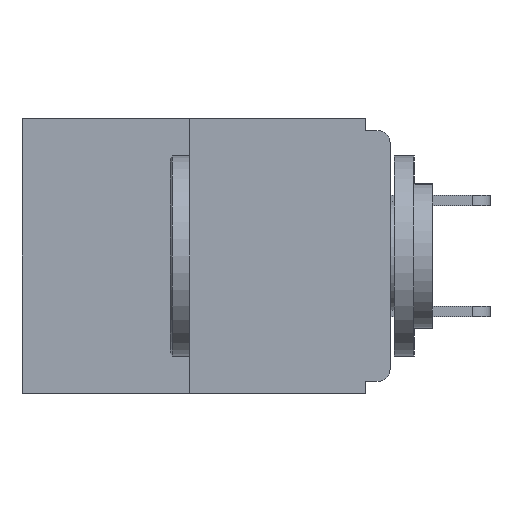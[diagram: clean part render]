
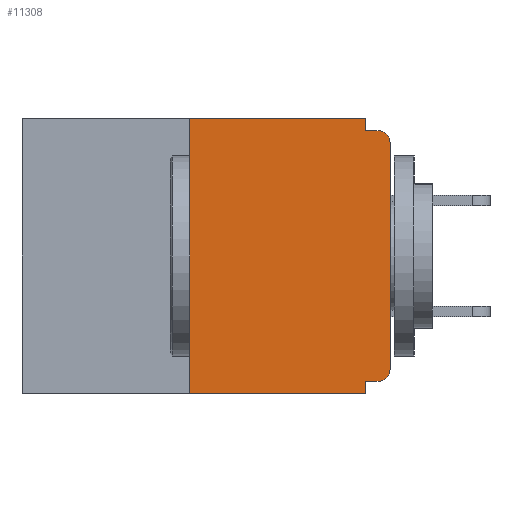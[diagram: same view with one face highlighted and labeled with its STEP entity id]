
A CAD part, left-side view. The second image highlights one B-rep face of the part: STEP entity #11308.
In plain terms, the highlighted planar face has unit normal (-1, 0, 0).
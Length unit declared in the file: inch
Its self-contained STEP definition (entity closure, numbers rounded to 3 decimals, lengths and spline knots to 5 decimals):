
#68 = CARTESIAN_POINT ( 'NONE',  ( 0., 0.25, 0. ) ) ;
#278 = CARTESIAN_POINT ( 'NONE',  ( 0., 0.031, -0.343 ) ) ;
#491 = DIRECTION ( 'NONE',  ( 0., 0., -1. ) ) ;
#777 = DIRECTION ( 'NONE',  ( 0., 0., -1. ) ) ;
#806 = LINE ( 'NONE', #7885, #6524 ) ;
#1189 = ORIENTED_EDGE ( 'NONE', *, *, #11605, .T. ) ;
#1291 = CARTESIAN_POINT ( 'NONE',  ( 0., 0.031, 0. ) ) ;
#1295 = CARTESIAN_POINT ( 'NONE',  ( 0., 0.031, -0.015 ) ) ;
#1330 = EDGE_CURVE ( 'NONE', #3055, #8899, #3673, .T. ) ;
#1400 = EDGE_CURVE ( 'NONE', #9018, #3647, #1813, .T. ) ;
#1755 = CARTESIAN_POINT ( 'NONE',  ( 0., 0.015, -0.328 ) ) ;
#1813 = LINE ( 'NONE', #68, #10220 ) ;
#2336 = DIRECTION ( 'NONE',  ( 0., 0., -1. ) ) ;
#2360 = AXIS2_PLACEMENT_3D ( 'NONE', #6239, #7247, #777 ) ;
#2524 = VERTEX_POINT ( 'NONE', #7561 ) ;
#2776 = CARTESIAN_POINT ( 'NONE',  ( 0., 0., -0.015 ) ) ;
#2872 = DIRECTION ( 'NONE',  ( 0., 1., 0. ) ) ;
#3055 = VERTEX_POINT ( 'NONE', #1295 ) ;
#3149 = CARTESIAN_POINT ( 'NONE',  ( 0., 0.031, 0. ) ) ;
#3382 = CIRCLE ( 'NONE', #3409, 0.015 ) ;
#3409 = AXIS2_PLACEMENT_3D ( 'NONE', #8807, #8959, #9700 ) ;
#3412 = ORIENTED_EDGE ( 'NONE', *, *, #9923, .F. ) ;
#3439 = VERTEX_POINT ( 'NONE', #278 ) ;
#3456 = CARTESIAN_POINT ( 'NONE',  ( 0., 0., -0.03 ) ) ;
#3516 = VECTOR ( 'NONE', #5304, 39.37008 ) ;
#3647 = VERTEX_POINT ( 'NONE', #10894 ) ;
#3673 = LINE ( 'NONE', #2776, #11531 ) ;
#3710 = CARTESIAN_POINT ( 'NONE',  ( 0., 0.25, -0.343 ) ) ;
#3763 = ORIENTED_EDGE ( 'NONE', *, *, #10119, .T. ) ;
#3972 = ORIENTED_EDGE ( 'NONE', *, *, #6391, .F. ) ;
#4036 = DIRECTION ( 'NONE',  ( 0., -1., 0. ) ) ;
#4500 = CIRCLE ( 'NONE', #2360, 0.015 ) ;
#5088 = VERTEX_POINT ( 'NONE', #3456 ) ;
#5304 = DIRECTION ( 'NONE',  ( 0., -1., 0. ) ) ;
#5388 = EDGE_CURVE ( 'NONE', #7239, #3055, #8576, .T. ) ;
#5801 = AXIS2_PLACEMENT_3D ( 'NONE', #10386, #6798, #491 ) ;
#5858 = EDGE_LOOP ( 'NONE', ( #3972, #7937, #9179, #3412, #8162, #1189, #6322, #3763, #10062, #10956 ) ) ;
#6231 = LINE ( 'NONE', #8011, #3516 ) ;
#6239 = CARTESIAN_POINT ( 'NONE',  ( 0., 0.015, -0.313 ) ) ;
#6322 = ORIENTED_EDGE ( 'NONE', *, *, #7130, .T. ) ;
#6391 = EDGE_CURVE ( 'NONE', #3647, #7239, #7022, .T. ) ;
#6411 = DIRECTION ( 'NONE',  ( 0., -1., 0. ) ) ;
#6478 = CARTESIAN_POINT ( 'NONE',  ( 0., 0., -0.328 ) ) ;
#6524 = VECTOR ( 'NONE', #2336, 39.37008 ) ;
#6798 = DIRECTION ( 'NONE',  ( 1., 0., 0. ) ) ;
#7022 = LINE ( 'NONE', #10374, #11603 ) ;
#7130 = EDGE_CURVE ( 'NONE', #2524, #5088, #10018, .T. ) ;
#7239 = VERTEX_POINT ( 'NONE', #3149 ) ;
#7247 = DIRECTION ( 'NONE',  ( -1., 0., 0. ) ) ;
#7517 = DIRECTION ( 'NONE',  ( 0., 0., 1. ) ) ;
#7561 = CARTESIAN_POINT ( 'NONE',  ( 0., 0., -0.313 ) ) ;
#7885 = CARTESIAN_POINT ( 'NONE',  ( 0., 0.031, -0.343 ) ) ;
#7937 = ORIENTED_EDGE ( 'NONE', *, *, #1400, .F. ) ;
#7970 = VERTEX_POINT ( 'NONE', #1755 ) ;
#8011 = CARTESIAN_POINT ( 'NONE',  ( 0., 0.46, -0.343 ) ) ;
#8162 = ORIENTED_EDGE ( 'NONE', *, *, #8728, .F. ) ;
#8291 = VECTOR ( 'NONE', #11348, 39.37008 ) ;
#8402 = LINE ( 'NONE', #6478, #9538 ) ;
#8576 = LINE ( 'NONE', #1291, #8291 ) ;
#8728 = EDGE_CURVE ( 'NONE', #7970, #10134, #8402, .T. ) ;
#8807 = CARTESIAN_POINT ( 'NONE',  ( 0., 0.015, -0.03 ) ) ;
#8899 = VERTEX_POINT ( 'NONE', #9856 ) ;
#8959 = DIRECTION ( 'NONE',  ( -1., 0., 0. ) ) ;
#9013 = DIRECTION ( 'NONE',  ( 0., 0., 1. ) ) ;
#9018 = VERTEX_POINT ( 'NONE', #3710 ) ;
#9179 = ORIENTED_EDGE ( 'NONE', *, *, #10037, .T. ) ;
#9313 = VECTOR ( 'NONE', #9013, 39.37008 ) ;
#9538 = VECTOR ( 'NONE', #2872, 39.37008 ) ;
#9700 = DIRECTION ( 'NONE',  ( 0., 0., -1. ) ) ;
#9856 = CARTESIAN_POINT ( 'NONE',  ( 0., 0.015, -0.015 ) ) ;
#9923 = EDGE_CURVE ( 'NONE', #10134, #3439, #806, .T. ) ;
#10018 = LINE ( 'NONE', #11730, #9313 ) ;
#10037 = EDGE_CURVE ( 'NONE', #9018, #3439, #6231, .T. ) ;
#10062 = ORIENTED_EDGE ( 'NONE', *, *, #1330, .F. ) ;
#10119 = EDGE_CURVE ( 'NONE', #5088, #8899, #3382, .T. ) ;
#10134 = VERTEX_POINT ( 'NONE', #10706 ) ;
#10190 = FACE_OUTER_BOUND ( 'NONE', #5858, .T. ) ;
#10220 = VECTOR ( 'NONE', #7517, 39.37008 ) ;
#10374 = CARTESIAN_POINT ( 'NONE',  ( 0., 0.46, 0. ) ) ;
#10386 = CARTESIAN_POINT ( 'NONE',  ( 0., 0.46, 0. ) ) ;
#10706 = CARTESIAN_POINT ( 'NONE',  ( 0., 0.031, -0.328 ) ) ;
#10894 = CARTESIAN_POINT ( 'NONE',  ( 0., 0.25, 0. ) ) ;
#10956 = ORIENTED_EDGE ( 'NONE', *, *, #5388, .F. ) ;
#11308 = ADVANCED_FACE ( 'NONE', ( #10190 ), #11390, .F. ) ;
#11348 = DIRECTION ( 'NONE',  ( 0., 0., -1. ) ) ;
#11390 = PLANE ( 'NONE',  #5801 ) ;
#11531 = VECTOR ( 'NONE', #6411, 39.37008 ) ;
#11603 = VECTOR ( 'NONE', #4036, 39.37008 ) ;
#11605 = EDGE_CURVE ( 'NONE', #7970, #2524, #4500, .T. ) ;
#11730 = CARTESIAN_POINT ( 'NONE',  ( 0., 0., 0. ) ) ;
